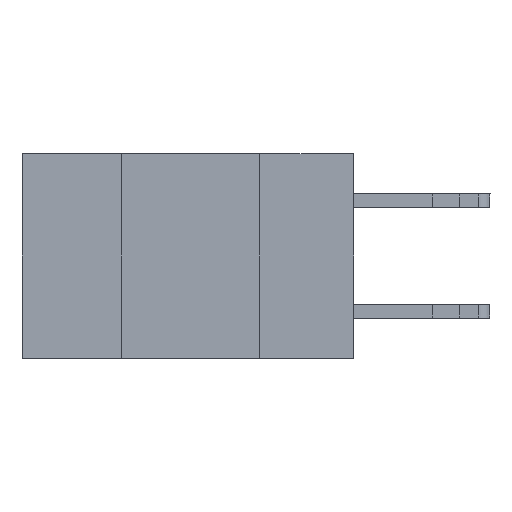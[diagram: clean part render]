
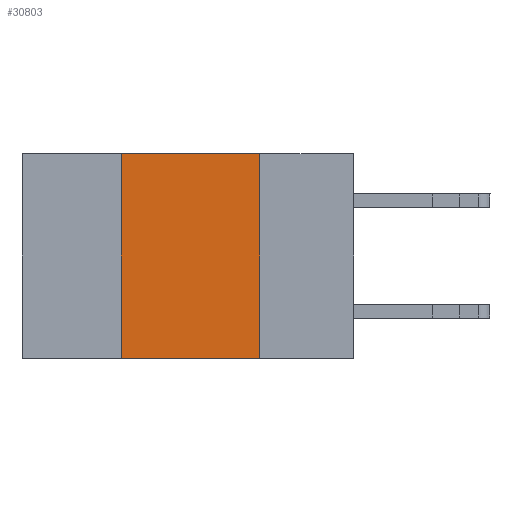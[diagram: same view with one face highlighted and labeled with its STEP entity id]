
A CAD part, left-side view. The second image highlights one B-rep face of the part: STEP entity #30803.
In plain terms, the highlighted planar face has unit normal (-1, 0, 0).
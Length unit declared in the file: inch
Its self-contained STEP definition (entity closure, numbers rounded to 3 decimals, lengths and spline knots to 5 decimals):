
#930 = CARTESIAN_POINT ( 'NONE',  ( 0., 0.42, -0.37 ) ) ;
#1690 = EDGE_CURVE ( 'NONE', #31894, #3877, #29986, .T. ) ;
#2600 = VECTOR ( 'NONE', #29962, 39.37008 ) ;
#3877 = VERTEX_POINT ( 'NONE', #6889 ) ;
#4013 = ORIENTED_EDGE ( 'NONE', *, *, #11030, .F. ) ;
#4337 = ORIENTED_EDGE ( 'NONE', *, *, #5823, .T. ) ;
#5823 = EDGE_CURVE ( 'NONE', #14279, #3877, #29633, .T. ) ;
#6889 = CARTESIAN_POINT ( 'NONE',  ( 0., 0.17, -0.37 ) ) ;
#7461 = FACE_OUTER_BOUND ( 'NONE', #21007, .T. ) ;
#7619 = DIRECTION ( 'NONE',  ( 1., 0., 0. ) ) ;
#9631 = AXIS2_PLACEMENT_3D ( 'NONE', #20005, #7619, #18535 ) ;
#10137 = DIRECTION ( 'NONE',  ( 0., 0., 1. ) ) ;
#11030 = EDGE_CURVE ( 'NONE', #14279, #14556, #17809, .T. ) ;
#13157 = ORIENTED_EDGE ( 'NONE', *, *, #1690, .F. ) ;
#13380 = DIRECTION ( 'NONE',  ( 0., 0., -1. ) ) ;
#14279 = VERTEX_POINT ( 'NONE', #930 ) ;
#14556 = VERTEX_POINT ( 'NONE', #22743 ) ;
#16249 = VECTOR ( 'NONE', #24159, 39.37008 ) ;
#16648 = CARTESIAN_POINT ( 'NONE',  ( 0., 0.6, 0. ) ) ;
#17396 = PLANE ( 'NONE',  #9631 ) ;
#17479 = CARTESIAN_POINT ( 'NONE',  ( 0., 0.42, 0. ) ) ;
#17706 = VECTOR ( 'NONE', #13380, 39.37008 ) ;
#17809 = LINE ( 'NONE', #17479, #19395 ) ;
#18535 = DIRECTION ( 'NONE',  ( 0., 0., -1. ) ) ;
#19395 = VECTOR ( 'NONE', #10137, 39.37008 ) ;
#20005 = CARTESIAN_POINT ( 'NONE',  ( 0., 0.6, 0. ) ) ;
#20075 = CARTESIAN_POINT ( 'NONE',  ( 0., 0.17, 0. ) ) ;
#21007 = EDGE_LOOP ( 'NONE', ( #13157, #23769, #4013, #4337 ) ) ;
#22743 = CARTESIAN_POINT ( 'NONE',  ( 0., 0.42, 0. ) ) ;
#23769 = ORIENTED_EDGE ( 'NONE', *, *, #25354, .F. ) ;
#24159 = DIRECTION ( 'NONE',  ( 0., -1., 0. ) ) ;
#25275 = CARTESIAN_POINT ( 'NONE',  ( 0., 0.6, -0.37 ) ) ;
#25354 = EDGE_CURVE ( 'NONE', #14556, #31894, #31606, .T. ) ;
#29598 = CARTESIAN_POINT ( 'NONE',  ( 0., 0.17, 0. ) ) ;
#29633 = LINE ( 'NONE', #25275, #2600 ) ;
#29962 = DIRECTION ( 'NONE',  ( 0., -1., 0. ) ) ;
#29986 = LINE ( 'NONE', #20075, #17706 ) ;
#30803 = ADVANCED_FACE ( 'NONE', ( #7461 ), #17396, .F. ) ;
#31606 = LINE ( 'NONE', #16648, #16249 ) ;
#31894 = VERTEX_POINT ( 'NONE', #29598 ) ;
